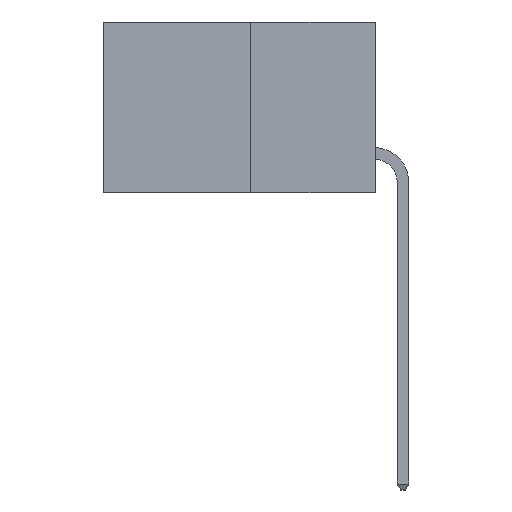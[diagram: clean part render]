
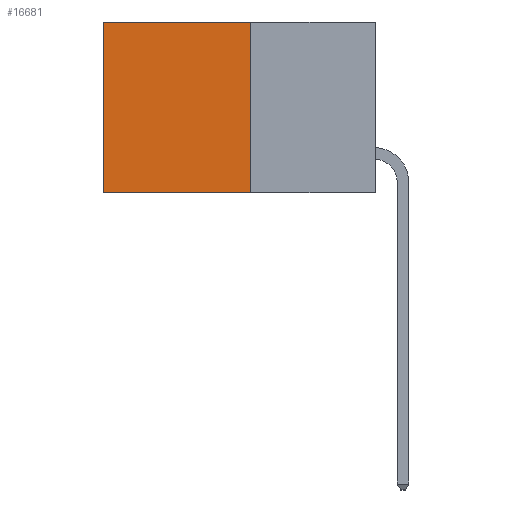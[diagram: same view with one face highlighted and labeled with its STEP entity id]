
A CAD part, left-side view. The second image highlights one B-rep face of the part: STEP entity #16681.
In plain terms, the highlighted planar face has unit normal (-1, 0, 0).
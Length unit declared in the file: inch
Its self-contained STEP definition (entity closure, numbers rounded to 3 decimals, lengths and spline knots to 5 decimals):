
#1628 = VERTEX_POINT ( 'NONE', #17924 ) ;
#3662 = LINE ( 'NONE', #17587, #16057 ) ;
#3854 = CARTESIAN_POINT ( 'NONE',  ( 0.277, 0.59, 0. ) ) ;
#3931 = FACE_OUTER_BOUND ( 'NONE', #18635, .T. ) ;
#4163 = VERTEX_POINT ( 'NONE', #3854 ) ;
#4705 = CARTESIAN_POINT ( 'NONE',  ( 0.277, 0.59, -0.37 ) ) ;
#4718 = CARTESIAN_POINT ( 'NONE',  ( 0.277, 0.27, 0. ) ) ;
#5227 = EDGE_CURVE ( 'NONE', #1628, #11792, #14764, .T. ) ;
#5422 = ORIENTED_EDGE ( 'NONE', *, *, #8145, .T. ) ;
#5563 = DIRECTION ( 'NONE',  ( 1., 0., 0. ) ) ;
#5793 = DIRECTION ( 'NONE',  ( 0., 0., -1. ) ) ;
#6038 = VERTEX_POINT ( 'NONE', #17479 ) ;
#6096 = EDGE_CURVE ( 'NONE', #6038, #1628, #3662, .T. ) ;
#7061 = VECTOR ( 'NONE', #18230, 39.37008 ) ;
#7573 = DIRECTION ( 'NONE',  ( 0., 0., -1. ) ) ;
#7927 = ORIENTED_EDGE ( 'NONE', *, *, #6096, .F. ) ;
#8145 = EDGE_CURVE ( 'NONE', #6038, #4163, #16766, .T. ) ;
#9594 = VECTOR ( 'NONE', #17619, 39.37008 ) ;
#11371 = CARTESIAN_POINT ( 'NONE',  ( 0.277, 0.27, -0.37 ) ) ;
#11792 = VERTEX_POINT ( 'NONE', #4705 ) ;
#12320 = EDGE_CURVE ( 'NONE', #4163, #11792, #17504, .T. ) ;
#12757 = PLANE ( 'NONE',  #18008 ) ;
#13060 = CARTESIAN_POINT ( 'NONE',  ( 0.277, 0.59, -0.37 ) ) ;
#13353 = VECTOR ( 'NONE', #5793, 39.37008 ) ;
#14708 = ORIENTED_EDGE ( 'NONE', *, *, #5227, .F. ) ;
#14764 = LINE ( 'NONE', #16835, #7061 ) ;
#15658 = DIRECTION ( 'NONE',  ( 0., 0., -1. ) ) ;
#16057 = VECTOR ( 'NONE', #7573, 39.37008 ) ;
#16681 = ADVANCED_FACE ( 'NONE', ( #3931 ), #12757, .F. ) ;
#16766 = LINE ( 'NONE', #4718, #9594 ) ;
#16835 = CARTESIAN_POINT ( 'NONE',  ( 0.277, 0.27, -0.37 ) ) ;
#17479 = CARTESIAN_POINT ( 'NONE',  ( 0.277, 0.27, 0. ) ) ;
#17504 = LINE ( 'NONE', #13060, #13353 ) ;
#17547 = ORIENTED_EDGE ( 'NONE', *, *, #12320, .T. ) ;
#17587 = CARTESIAN_POINT ( 'NONE',  ( 0.277, 0.27, -0.37 ) ) ;
#17619 = DIRECTION ( 'NONE',  ( 0., 1., 0. ) ) ;
#17924 = CARTESIAN_POINT ( 'NONE',  ( 0.277, 0.27, -0.37 ) ) ;
#18008 = AXIS2_PLACEMENT_3D ( 'NONE', #11371, #5563, #15658 ) ;
#18230 = DIRECTION ( 'NONE',  ( 0., 1., 0. ) ) ;
#18635 = EDGE_LOOP ( 'NONE', ( #17547, #14708, #7927, #5422 ) ) ;
